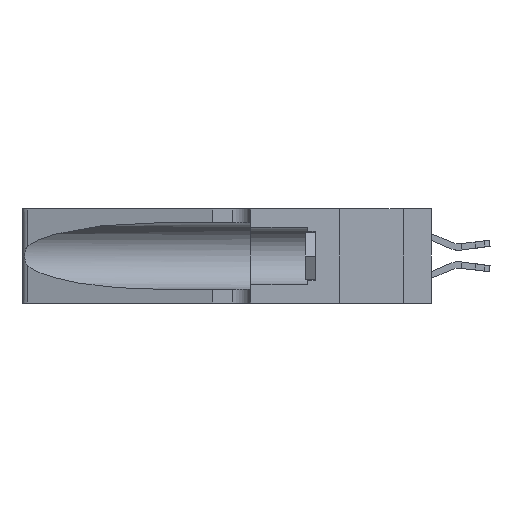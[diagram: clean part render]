
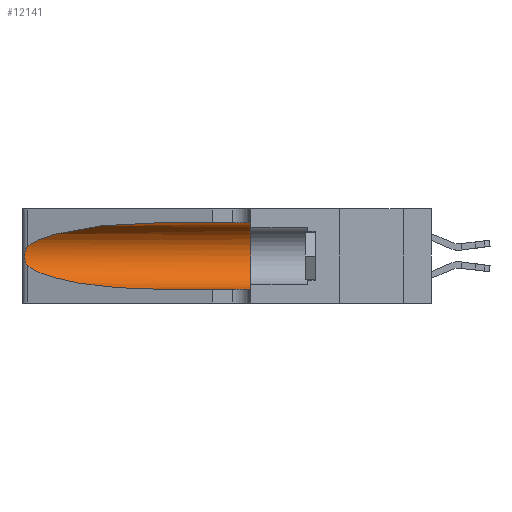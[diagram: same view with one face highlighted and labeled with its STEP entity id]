
A CAD part, left-side view. The second image highlights one B-rep face of the part: STEP entity #12141.
In plain terms, the highlighted cylindrical face has radius 3.308 mm (diameter 6.617 mm), a partial arc.
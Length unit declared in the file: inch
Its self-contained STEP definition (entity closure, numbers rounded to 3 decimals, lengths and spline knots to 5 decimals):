
#577 = CARTESIAN_POINT ( 'NONE',  ( 0.18966, 0.96281, 0.31525 ) ) ;
#794 = EDGE_CURVE ( 'NONE', #1521, #21521, #10723, .T. ) ;
#1521 = VERTEX_POINT ( 'NONE', #20453 ) ;
#2204 = CARTESIAN_POINT ( 'NONE',  ( 0.25487, 1.22718, 0.14631 ) ) ;
#2258 = DIRECTION ( 'NONE',  ( 0., -1., 0. ) ) ;
#2472 = EDGE_CURVE ( 'NONE', #5627, #15865, #15963, .T. ) ;
#2962 = ORIENTED_EDGE ( 'NONE', *, *, #2472, .T. ) ;
#3986 = CARTESIAN_POINT ( 'NONE',  ( 0.25487, 1.22718, 0.22369 ) ) ;
#4049 = DIRECTION ( 'NONE',  ( 0., 0., -1. ) ) ;
#4207 = CARTESIAN_POINT ( 'NONE',  ( 0.1305, 1.61858, 0.185 ) ) ;
#4760 = DIRECTION ( 'NONE',  ( 0., 1., 0. ) ) ;
#4998 = CARTESIAN_POINT ( 'NONE',  ( 0.1305, 0.35, 0.31525 ) ) ;
#5123 = VECTOR ( 'NONE', #2258, 39.37008 ) ;
#5135 = EDGE_CURVE ( 'NONE', #5627, #10241, #19464, .T. ) ;
#5627 = VERTEX_POINT ( 'NONE', #6004 ) ;
#5700 = CARTESIAN_POINT ( 'NONE',  ( 0.26075, 1.23896, 0.178 ) ) ;
#6004 = CARTESIAN_POINT ( 'NONE',  ( 0.1305, 0.72297, 0.31525 ) ) ;
#6222 = CARTESIAN_POINT ( 'NONE',  ( 0.1305, 1.61858, 0.05475 ) ) ;
#6707 = ORIENTED_EDGE ( 'NONE', *, *, #5135, .F. ) ;
#8344 = ORIENTED_EDGE ( 'NONE', *, *, #16869, .F. ) ;
#8932 = AXIS2_PLACEMENT_3D ( 'NONE', #4207, #18189, #4049 ) ;
#8942 = CARTESIAN_POINT ( 'NONE',  ( 0.25487, 1.22718, 0.22369 ) ) ;
#9077 = CARTESIAN_POINT ( 'NONE',  ( 0.25856, 1.23593, 0.16098 ) ) ;
#9301 = ORIENTED_EDGE ( 'NONE', *, *, #13351, .T. ) ;
#10183 = AXIS2_PLACEMENT_3D ( 'NONE', #13770, #4760, #15764 ) ;
#10241 = VERTEX_POINT ( 'NONE', #4998 ) ;
#10723 =( BOUNDED_CURVE ( )  B_SPLINE_CURVE ( 3, ( #12484, #14316, #21640, #12561 ),
 .UNSPECIFIED., .F., .T. ) 
 B_SPLINE_CURVE_WITH_KNOTS ( ( 4, 4 ),
 ( 3.44316, 4.71239 ),
 .UNSPECIFIED. ) 
 CURVE ( )  GEOMETRIC_REPRESENTATION_ITEM ( )  RATIONAL_B_SPLINE_CURVE ( ( 1., 0.87, 0.87, 1. ) ) 
 REPRESENTATION_ITEM ( '' )  );
#10928 = CARTESIAN_POINT ( 'NONE',  ( 0.1305, 1.61858, 0.31525 ) ) ;
#10953 = CARTESIAN_POINT ( 'NONE',  ( 0.25789, 1.23486, 0.15765 ) ) ;
#11104 = CARTESIAN_POINT ( 'NONE',  ( 0.25639, 1.23186, 0.15144 ) ) ;
#11138 = LINE ( 'NONE', #6222, #16232 ) ;
#11540 = EDGE_CURVE ( 'NONE', #21521, #20373, #11138, .T. ) ;
#11689 = CYLINDRICAL_SURFACE ( 'NONE', #8932, 0.13025 ) ;
#12141 = ADVANCED_FACE ( 'NONE', ( #22433 ), #11689, .F. ) ;
#12484 = CARTESIAN_POINT ( 'NONE',  ( 0.25487, 1.22718, 0.14631 ) ) ;
#12561 = CARTESIAN_POINT ( 'NONE',  ( 0.1305, 0.72297, 0.05475 ) ) ;
#12671 = CARTESIAN_POINT ( 'NONE',  ( 0.25555, 1.22994, 0.2215 ) ) ;
#13351 = EDGE_CURVE ( 'NONE', #15865, #1521, #22311, .T. ) ;
#13770 = CARTESIAN_POINT ( 'NONE',  ( 0.1305, 0.35, 0.185 ) ) ;
#14163 = ORIENTED_EDGE ( 'NONE', *, *, #11540, .T. ) ;
#14316 = CARTESIAN_POINT ( 'NONE',  ( 0.2373, 1.15595, 0.08982 ) ) ;
#14412 = CARTESIAN_POINT ( 'NONE',  ( 0.25787, 1.23484, 0.2124 ) ) ;
#14488 = CARTESIAN_POINT ( 'NONE',  ( 0.26075, 1.23896, 0.19203 ) ) ;
#14565 = CARTESIAN_POINT ( 'NONE',  ( 0.25639, 1.23184, 0.21858 ) ) ;
#14653 = CARTESIAN_POINT ( 'NONE',  ( 0.26018, 1.23835, 0.19895 ) ) ;
#14797 = ORIENTED_EDGE ( 'NONE', *, *, #794, .T. ) ;
#15762 = EDGE_LOOP ( 'NONE', ( #2962, #9301, #14797, #14163, #8344, #6707 ) ) ;
#15764 = DIRECTION ( 'NONE',  ( 0., 0., 1. ) ) ;
#15865 = VERTEX_POINT ( 'NONE', #8942 ) ;
#15963 =( BOUNDED_CURVE ( )  B_SPLINE_CURVE ( 3, ( #22054, #577, #18131, #18281 ),
 .UNSPECIFIED., .F., .F. ) 
 B_SPLINE_CURVE_WITH_KNOTS ( ( 4, 4 ),
 ( 1.5708, 2.84003 ),
 .UNSPECIFIED. ) 
 CURVE ( )  GEOMETRIC_REPRESENTATION_ITEM ( )  RATIONAL_B_SPLINE_CURVE ( ( 1., 0.87, 0.87, 1. ) ) 
 REPRESENTATION_ITEM ( '' )  );
#16232 = VECTOR ( 'NONE', #22506, 39.37008 ) ;
#16586 = CARTESIAN_POINT ( 'NONE',  ( 0.25854, 1.2359, 0.20912 ) ) ;
#16869 = EDGE_CURVE ( 'NONE', #10241, #20373, #19977, .T. ) ;
#17419 = CARTESIAN_POINT ( 'NONE',  ( 0.1305, 0.35, 0.05475 ) ) ;
#18131 = CARTESIAN_POINT ( 'NONE',  ( 0.2373, 1.15595, 0.28018 ) ) ;
#18189 = DIRECTION ( 'NONE',  ( 0., -1., 0. ) ) ;
#18281 = CARTESIAN_POINT ( 'NONE',  ( 0.25487, 1.22718, 0.22369 ) ) ;
#18369 = CARTESIAN_POINT ( 'NONE',  ( 0.1305, 0.72297, 0.05475 ) ) ;
#19464 = LINE ( 'NONE', #10928, #5123 ) ;
#19938 = CARTESIAN_POINT ( 'NONE',  ( 0.26017, 1.23833, 0.17102 ) ) ;
#19977 = CIRCLE ( 'NONE', #10183, 0.13025 ) ;
#20373 = VERTEX_POINT ( 'NONE', #17419 ) ;
#20453 = CARTESIAN_POINT ( 'NONE',  ( 0.25487, 1.22718, 0.14631 ) ) ;
#21521 = VERTEX_POINT ( 'NONE', #18369 ) ;
#21640 = CARTESIAN_POINT ( 'NONE',  ( 0.18966, 0.96281, 0.05475 ) ) ;
#21743 = CARTESIAN_POINT ( 'NONE',  ( 0.25555, 1.22993, 0.14849 ) ) ;
#22054 = CARTESIAN_POINT ( 'NONE',  ( 0.1305, 0.72297, 0.31525 ) ) ;
#22311 = B_SPLINE_CURVE_WITH_KNOTS ( 'NONE', 3,
 ( #3986, #12671, #14565, #14412, #16586, #14653, #14488, #5700, #19938, #9077, #10953, #11104, #21743, #2204 ),
 .UNSPECIFIED., .F., .F.,
 ( 4, 2, 2, 2, 2, 2, 4 ),
 ( 0., 0.00027, 0.00053, 0.00107, 0.0016, 0.00187, 0.00214 ),
 .UNSPECIFIED. ) ;
#22433 = FACE_OUTER_BOUND ( 'NONE', #15762, .T. ) ;
#22506 = DIRECTION ( 'NONE',  ( 0., -1., 0. ) ) ;
